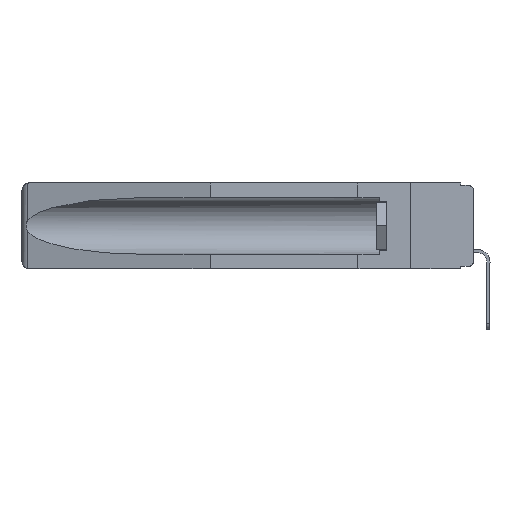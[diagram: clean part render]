
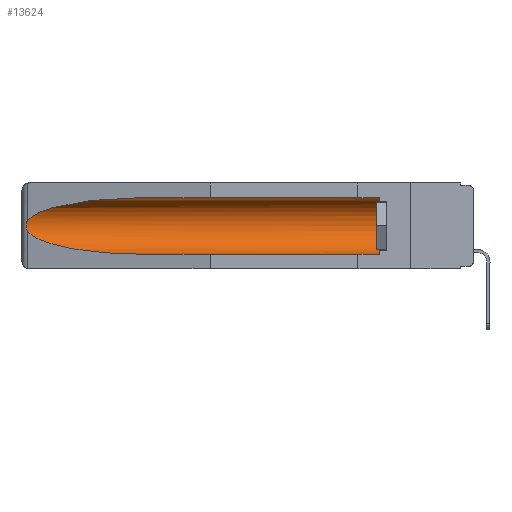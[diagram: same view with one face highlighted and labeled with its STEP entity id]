
A CAD part, left-side view. The second image highlights one B-rep face of the part: STEP entity #13624.
In plain terms, the highlighted cylindrical face has radius 2.857 mm (diameter 5.715 mm), a partial arc.
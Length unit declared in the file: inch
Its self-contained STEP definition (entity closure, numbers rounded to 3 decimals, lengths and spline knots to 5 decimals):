
#373 = ORIENTED_EDGE ( 'NONE', *, *, #11601, .T. ) ;
#809 = CIRCLE ( 'NONE', #16272, 0.1125 ) ;
#1000 = CARTESIAN_POINT ( 'NONE',  ( 0.26537, 1.52718, -0.19328 ) ) ;
#1082 = ORIENTED_EDGE ( 'NONE', *, *, #10187, .T. ) ;
#1238 = CARTESIAN_POINT ( 'NONE',  ( 0.155, 1.07973, -0.284 ) ) ;
#1258 = CARTESIAN_POINT ( 'NONE',  ( 0.26597, 1.52961, -0.15275 ) ) ;
#1287 = VECTOR ( 'NONE', #11947, 39.37008 ) ;
#1509 = ORIENTED_EDGE ( 'NONE', *, *, #6407, .T. ) ;
#1621 = DIRECTION ( 'NONE',  ( 0., 0., 1. ) ) ;
#1756 = CARTESIAN_POINT ( 'NONE',  ( 0.155, 1.07973, -0.284 ) ) ;
#1843 = VERTEX_POINT ( 'NONE', #13716 ) ;
#2371 = AXIS2_PLACEMENT_3D ( 'NONE', #5383, #11782, #1621 ) ;
#2836 = LINE ( 'NONE', #15864, #10125 ) ;
#3393 = CARTESIAN_POINT ( 'NONE',  ( 0.155, -0.30754, -0.059 ) ) ;
#3789 = CARTESIAN_POINT ( 'NONE',  ( 0.155, 1.07973, -0.059 ) ) ;
#3882 = CARTESIAN_POINT ( 'NONE',  ( 0.155, 0.126, -0.059 ) ) ;
#4436 = VERTEX_POINT ( 'NONE', #3789 ) ;
#4525 = DIRECTION ( 'NONE',  ( 0., 0., 1. ) ) ;
#4914 = CARTESIAN_POINT ( 'NONE',  ( 0.21114, 1.30732, -0.284 ) ) ;
#5205 = ORIENTED_EDGE ( 'NONE', *, *, #17698, .T. ) ;
#5383 = CARTESIAN_POINT ( 'NONE',  ( 0.155, -0.30754, -0.1715 ) ) ;
#6407 = EDGE_CURVE ( 'NONE', #11923, #9707, #16441, .T. ) ;
#6518 = CARTESIAN_POINT ( 'NONE',  ( 0.25451, 1.48313, -0.24835 ) ) ;
#6595 = ORIENTED_EDGE ( 'NONE', *, *, #17500, .F. ) ;
#7056 = CARTESIAN_POINT ( 'NONE',  ( 0.2675, 1.53308, -0.16763 ) ) ;
#8433 = CARTESIAN_POINT ( 'NONE',  ( 0.25451, 1.48313, -0.09465 ) ) ;
#8734 = DIRECTION ( 'NONE',  ( 0., 1., 0. ) ) ;
#8873 = CARTESIAN_POINT ( 'NONE',  ( 0.26537, 1.52718, -0.14972 ) ) ;
#9117 = LINE ( 'NONE', #3393, #1287 ) ;
#9288 =( BOUNDED_CURVE ( )  B_SPLINE_CURVE ( 3, ( #11284, #15660, #8433, #14239 ),
 .UNSPECIFIED., .F., .F. ) 
 B_SPLINE_CURVE_WITH_KNOTS ( ( 4, 4 ),
 ( 4.71239, 6.08839 ),
 .UNSPECIFIED. ) 
 CURVE ( )  GEOMETRIC_REPRESENTATION_ITEM ( )  RATIONAL_B_SPLINE_CURVE ( ( 1., 0.848, 0.848, 1. ) ) 
 REPRESENTATION_ITEM ( '' )  );
#9371 = CARTESIAN_POINT ( 'NONE',  ( 0.26537, 1.52718, -0.19328 ) ) ;
#9632 = CARTESIAN_POINT ( 'NONE',  ( 0.26654, 1.53092, -0.15636 ) ) ;
#9707 = VERTEX_POINT ( 'NONE', #1238 ) ;
#10125 = VECTOR ( 'NONE', #8734, 39.37008 ) ;
#10187 = EDGE_CURVE ( 'NONE', #4436, #16616, #9288, .T. ) ;
#10506 = DIRECTION ( 'NONE',  ( 0., -1., 0. ) ) ;
#11218 = ORIENTED_EDGE ( 'NONE', *, *, #12380, .T. ) ;
#11237 = VERTEX_POINT ( 'NONE', #3882 ) ;
#11284 = CARTESIAN_POINT ( 'NONE',  ( 0.155, 1.07973, -0.059 ) ) ;
#11601 = EDGE_CURVE ( 'NONE', #1843, #11237, #809, .T. ) ;
#11782 = DIRECTION ( 'NONE',  ( 0., 1., 0. ) ) ;
#11923 = VERTEX_POINT ( 'NONE', #1000 ) ;
#11947 = DIRECTION ( 'NONE',  ( 0., 1., 0. ) ) ;
#12380 = EDGE_CURVE ( 'NONE', #16616, #11923, #15128, .T. ) ;
#12561 = CARTESIAN_POINT ( 'NONE',  ( 0.2675, 1.53308, -0.17534 ) ) ;
#12937 = CARTESIAN_POINT ( 'NONE',  ( 0.26537, 1.52718, -0.19328 ) ) ;
#13624 = ADVANCED_FACE ( 'NONE', ( #15796 ), #18358, .F. ) ;
#13716 = CARTESIAN_POINT ( 'NONE',  ( 0.155, 0.126, -0.284 ) ) ;
#14239 = CARTESIAN_POINT ( 'NONE',  ( 0.26537, 1.52718, -0.14972 ) ) ;
#14276 = CARTESIAN_POINT ( 'NONE',  ( 0.26537, 1.52718, -0.14972 ) ) ;
#14638 = CARTESIAN_POINT ( 'NONE',  ( 0.26655, 1.53094, -0.18657 ) ) ;
#15128 = B_SPLINE_CURVE_WITH_KNOTS ( 'NONE', 3,
 ( #14276, #1258, #9632, #15417, #7056, #12561, #18353, #14638, #17475, #12937 ),
 .UNSPECIFIED., .F., .F.,
 ( 4, 2, 2, 2, 4 ),
 ( 0., 0.00029, 0.00058, 0.00087, 0.00117 ),
 .UNSPECIFIED. ) ;
#15417 = CARTESIAN_POINT ( 'NONE',  ( 0.2673, 1.5327, -0.16383 ) ) ;
#15660 = CARTESIAN_POINT ( 'NONE',  ( 0.21114, 1.30732, -0.059 ) ) ;
#15796 = FACE_OUTER_BOUND ( 'NONE', #17635, .T. ) ;
#15864 = CARTESIAN_POINT ( 'NONE',  ( 0.155, -0.30754, -0.284 ) ) ;
#16272 = AXIS2_PLACEMENT_3D ( 'NONE', #17524, #10506, #4525 ) ;
#16441 =( BOUNDED_CURVE ( )  B_SPLINE_CURVE ( 3, ( #9371, #6518, #4914, #1756 ),
 .UNSPECIFIED., .F., .F. ) 
 B_SPLINE_CURVE_WITH_KNOTS ( ( 4, 4 ),
 ( 0.1948, 1.5708 ),
 .UNSPECIFIED. ) 
 CURVE ( )  GEOMETRIC_REPRESENTATION_ITEM ( )  RATIONAL_B_SPLINE_CURVE ( ( 1., 0.848, 0.848, 1. ) ) 
 REPRESENTATION_ITEM ( '' )  );
#16616 = VERTEX_POINT ( 'NONE', #8873 ) ;
#17475 = CARTESIAN_POINT ( 'NONE',  ( 0.26597, 1.5296, -0.19026 ) ) ;
#17500 = EDGE_CURVE ( 'NONE', #1843, #9707, #2836, .T. ) ;
#17524 = CARTESIAN_POINT ( 'NONE',  ( 0.155, 0.126, -0.1715 ) ) ;
#17635 = EDGE_LOOP ( 'NONE', ( #1082, #11218, #1509, #6595, #373, #5205 ) ) ;
#17698 = EDGE_CURVE ( 'NONE', #11237, #4436, #9117, .T. ) ;
#18353 = CARTESIAN_POINT ( 'NONE',  ( 0.2673, 1.53269, -0.17917 ) ) ;
#18358 = CYLINDRICAL_SURFACE ( 'NONE', #2371, 0.1125 ) ;
